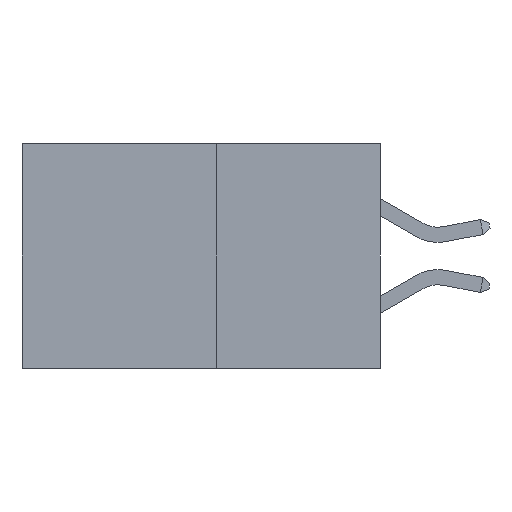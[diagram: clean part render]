
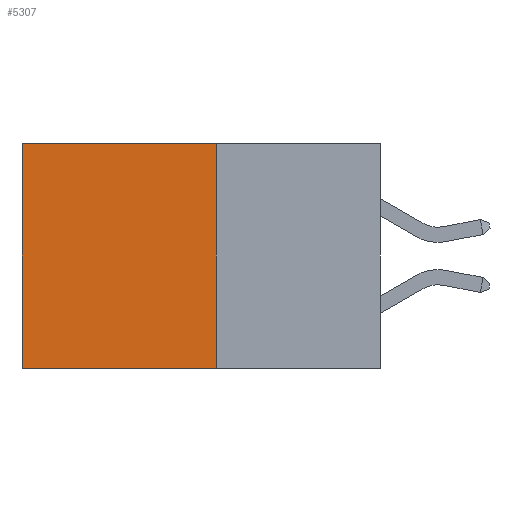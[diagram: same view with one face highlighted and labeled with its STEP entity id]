
A CAD part, left-side view. The second image highlights one B-rep face of the part: STEP entity #5307.
In plain terms, the highlighted planar face has unit normal (-1, 0, 0).
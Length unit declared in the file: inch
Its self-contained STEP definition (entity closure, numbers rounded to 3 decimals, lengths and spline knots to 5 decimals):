
#627 = AXIS2_PLACEMENT_3D ( 'NONE', #7026, #5690, #4533 ) ;
#628 = CARTESIAN_POINT ( 'NONE',  ( 0.277, 0.27, -0.37 ) ) ;
#899 = DIRECTION ( 'NONE',  ( 0., 0., -1. ) ) ;
#1187 = VERTEX_POINT ( 'NONE', #1389 ) ;
#1389 = CARTESIAN_POINT ( 'NONE',  ( 0.277, 0.59, 0. ) ) ;
#1394 = EDGE_CURVE ( 'NONE', #5352, #1187, #8908, .T. ) ;
#1502 = CARTESIAN_POINT ( 'NONE',  ( 0.277, 0.27, -0.37 ) ) ;
#1642 = VECTOR ( 'NONE', #4171, 39.37008 ) ;
#1980 = LINE ( 'NONE', #628, #3729 ) ;
#2210 = LINE ( 'NONE', #1502, #4183 ) ;
#2933 = DIRECTION ( 'NONE',  ( 0., 1., 0. ) ) ;
#2955 = VERTEX_POINT ( 'NONE', #4905 ) ;
#3614 = LINE ( 'NONE', #4873, #1642 ) ;
#3729 = VECTOR ( 'NONE', #899, 39.37008 ) ;
#3963 = EDGE_CURVE ( 'NONE', #1187, #2955, #3614, .T. ) ;
#4171 = DIRECTION ( 'NONE',  ( 0., 0., -1. ) ) ;
#4183 = VECTOR ( 'NONE', #2933, 39.37008 ) ;
#4386 = FACE_OUTER_BOUND ( 'NONE', #5154, .T. ) ;
#4498 = EDGE_CURVE ( 'NONE', #6825, #2955, #2210, .T. ) ;
#4533 = DIRECTION ( 'NONE',  ( 0., 0., -1. ) ) ;
#4873 = CARTESIAN_POINT ( 'NONE',  ( 0.277, 0.59, -0.37 ) ) ;
#4905 = CARTESIAN_POINT ( 'NONE',  ( 0.277, 0.59, -0.37 ) ) ;
#5154 = EDGE_LOOP ( 'NONE', ( #9486, #9492, #9509, #9521 ) ) ;
#5307 = ADVANCED_FACE ( 'NONE', ( #4386 ), #8047, .F. ) ;
#5352 = VERTEX_POINT ( 'NONE', #6113 ) ;
#5457 = DIRECTION ( 'NONE',  ( 0., 1., 0. ) ) ;
#5690 = DIRECTION ( 'NONE',  ( 1., 0., 0. ) ) ;
#6113 = CARTESIAN_POINT ( 'NONE',  ( 0.277, 0.27, 0. ) ) ;
#6456 = CARTESIAN_POINT ( 'NONE',  ( 0.277, 0.27, 0. ) ) ;
#6825 = VERTEX_POINT ( 'NONE', #9087 ) ;
#7026 = CARTESIAN_POINT ( 'NONE',  ( 0.277, 0.27, -0.37 ) ) ;
#8047 = PLANE ( 'NONE',  #627 ) ;
#8271 = EDGE_CURVE ( 'NONE', #5352, #6825, #1980, .T. ) ;
#8678 = VECTOR ( 'NONE', #5457, 39.37008 ) ;
#8908 = LINE ( 'NONE', #6456, #8678 ) ;
#9087 = CARTESIAN_POINT ( 'NONE',  ( 0.277, 0.27, -0.37 ) ) ;
#9486 = ORIENTED_EDGE ( 'NONE', *, *, #3963, .T. ) ;
#9492 = ORIENTED_EDGE ( 'NONE', *, *, #4498, .F. ) ;
#9509 = ORIENTED_EDGE ( 'NONE', *, *, #8271, .F. ) ;
#9521 = ORIENTED_EDGE ( 'NONE', *, *, #1394, .T. ) ;
